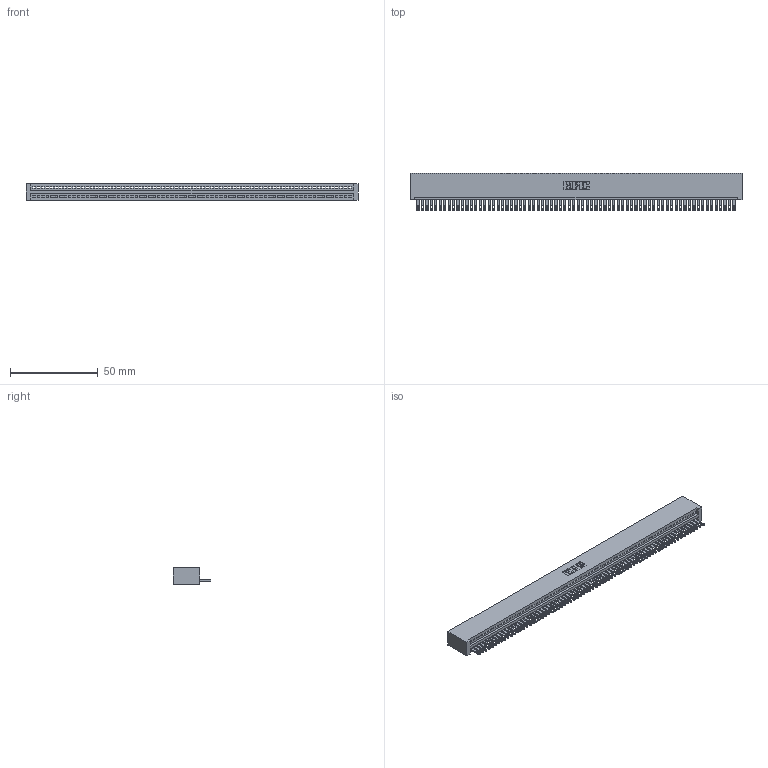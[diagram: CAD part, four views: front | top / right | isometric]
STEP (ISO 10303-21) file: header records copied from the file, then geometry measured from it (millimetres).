
FILE_DESCRIPTION (( 'STEP AP203' ), '1' );
FILE_NAME ('345-072-500-101.STEP', '2019-10-13T01:40:33', ( '' ), ( '' ), 'SwSTEP 2.0', 'SolidWorks 2016', '' );
FILE_SCHEMA (( 'CONFIG_CONTROL_DESIGN' ));
Length unit declared in the file: inch
Products named in the file (3): 345 Part_No Mounting Lugs; 345-292-001_345-293-100; 345-072-500-101
Assembly tree (73 placements, depth 2):
  345-072-500-101
    345 Part_No Mounting Lugs
    345-292-001_345-293-100  x72
Bounding box: 189.48 x 21.51 x 9.4 mm (x, y, z)
Volume: 18872.1 mm3; surface area: 25838.8 mm2
Topology: 73 solids, 73 shells, 4006 faces, 12413 edges, 8274 vertices
Faces by surface type: plane 2524, cylinder 1482
Entity records: 49803 total; most frequent: ORIENTED_EDGE 8638, CARTESIAN_POINT 8632, DIRECTION 7491, EDGE_CURVE 4319, LINE 3903, VECTOR 3903, VERTEX_POINT 2878, AXIS2_PLACEMENT_3D 1794
